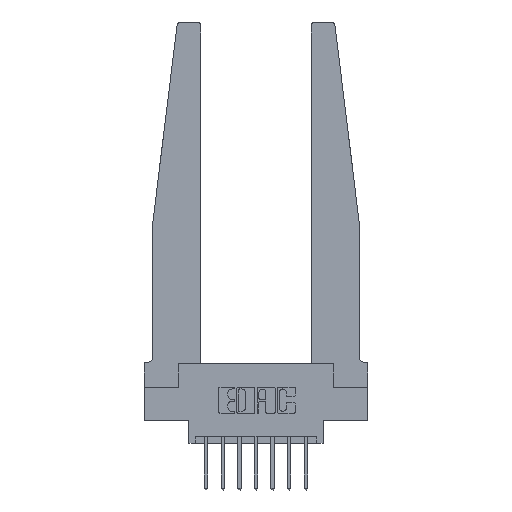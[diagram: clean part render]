
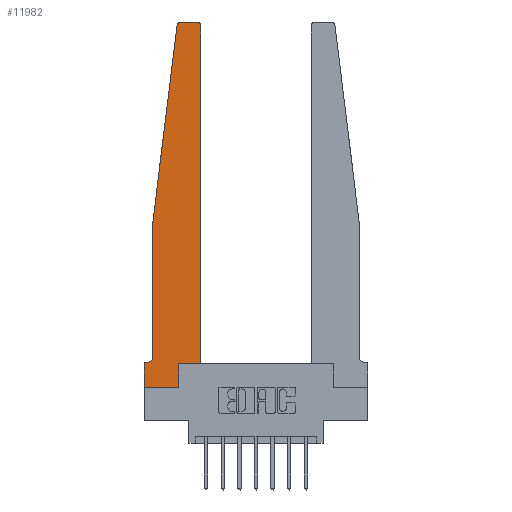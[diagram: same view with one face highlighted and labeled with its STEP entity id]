
A CAD part, top view. The second image highlights one B-rep face of the part: STEP entity #11982.
In plain terms, the highlighted planar face has unit normal (0, 0, 1).
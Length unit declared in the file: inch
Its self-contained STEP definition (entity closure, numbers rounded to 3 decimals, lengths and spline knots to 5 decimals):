
#76 = VERTEX_POINT ( 'NONE', #4507 ) ;
#304 = EDGE_CURVE ( 'NONE', #1373, #2586, #9048, .T. ) ;
#507 = CARTESIAN_POINT ( 'NONE',  ( 0., 0.1875, 0.37 ) ) ;
#565 = ORIENTED_EDGE ( 'NONE', *, *, #2735, .T. ) ;
#770 = CARTESIAN_POINT ( 'NONE',  ( 0.425, 0.18, 0.37 ) ) ;
#789 = LINE ( 'NONE', #14413, #3189 ) ;
#1053 = CARTESIAN_POINT ( 'NONE',  ( 0.065, 0.1875, 0.37 ) ) ;
#1319 = AXIS2_PLACEMENT_3D ( 'NONE', #11494, #12881, #6173 ) ;
#1373 = VERTEX_POINT ( 'NONE', #14378 ) ;
#1492 = EDGE_CURVE ( 'NONE', #8797, #5418, #789, .T. ) ;
#1594 = CARTESIAN_POINT ( 'NONE',  ( 0.2605, 0.18, 0.37 ) ) ;
#1624 = CARTESIAN_POINT ( 'NONE',  ( 0., 0., 0.37 ) ) ;
#1711 = VERTEX_POINT ( 'NONE', #5702 ) ;
#1904 = VECTOR ( 'NONE', #4447, 39.37008 ) ;
#2036 = CARTESIAN_POINT ( 'NONE',  ( 0.395, 2.72, 0.37 ) ) ;
#2131 = EDGE_CURVE ( 'NONE', #6667, #3614, #11939, .T. ) ;
#2146 = LINE ( 'NONE', #7879, #3322 ) ;
#2527 = EDGE_LOOP ( 'NONE', ( #3956, #9566, #7385, #7978, #10287, #3680, #4014, #5228, #5180, #12531, #565, #14125 ) ) ;
#2586 = VERTEX_POINT ( 'NONE', #6468 ) ;
#2670 = CARTESIAN_POINT ( 'NONE',  ( 0.2605, 0.18, 0.37 ) ) ;
#2689 = CARTESIAN_POINT ( 'NONE',  ( 0.015, 0.2375, 0.37 ) ) ;
#2735 = EDGE_CURVE ( 'NONE', #5418, #1373, #2146, .T. ) ;
#2906 = VECTOR ( 'NONE', #9753, 39.37008 ) ;
#2963 = LINE ( 'NONE', #8903, #6334 ) ;
#3189 = VECTOR ( 'NONE', #9775, 39.37008 ) ;
#3256 = VERTEX_POINT ( 'NONE', #13943 ) ;
#3322 = VECTOR ( 'NONE', #12367, 39.37008 ) ;
#3614 = VERTEX_POINT ( 'NONE', #11118 ) ;
#3680 = ORIENTED_EDGE ( 'NONE', *, *, #8718, .T. ) ;
#3815 = AXIS2_PLACEMENT_3D ( 'NONE', #2036, #5167, #5092 ) ;
#3956 = ORIENTED_EDGE ( 'NONE', *, *, #4637, .T. ) ;
#4014 = ORIENTED_EDGE ( 'NONE', *, *, #5359, .T. ) ;
#4137 = VECTOR ( 'NONE', #13999, 39.37008 ) ;
#4188 = CARTESIAN_POINT ( 'NONE',  ( 0.065, 0.2375, 0.37 ) ) ;
#4447 = DIRECTION ( 'NONE',  ( -1., 0., 0. ) ) ;
#4507 = CARTESIAN_POINT ( 'NONE',  ( 0., 0.1875, 0.37 ) ) ;
#4637 = EDGE_CURVE ( 'NONE', #2586, #7283, #12360, .T. ) ;
#5048 = DIRECTION ( 'NONE',  ( 0., 0., 1. ) ) ;
#5092 = DIRECTION ( 'NONE',  ( 1., 0., 0. ) ) ;
#5167 = DIRECTION ( 'NONE',  ( 0., 0., 1. ) ) ;
#5180 = ORIENTED_EDGE ( 'NONE', *, *, #8181, .T. ) ;
#5228 = ORIENTED_EDGE ( 'NONE', *, *, #7321, .T. ) ;
#5359 = EDGE_CURVE ( 'NONE', #76, #1711, #13141, .T. ) ;
#5418 = VERTEX_POINT ( 'NONE', #770 ) ;
#5437 = CARTESIAN_POINT ( 'NONE',  ( 0.2605, 0., 0.37 ) ) ;
#5702 = CARTESIAN_POINT ( 'NONE',  ( 0., 0., 0.37 ) ) ;
#5819 = VERTEX_POINT ( 'NONE', #5437 ) ;
#5835 = VECTOR ( 'NONE', #14401, 39.37008 ) ;
#5953 = CARTESIAN_POINT ( 'NONE',  ( 0.27653, 2.75, 0.37 ) ) ;
#6067 = CIRCLE ( 'NONE', #1319, 0.03 ) ;
#6136 = DIRECTION ( 'NONE',  ( 0., 1., 0. ) ) ;
#6159 = FACE_OUTER_BOUND ( 'NONE', #2527, .T. ) ;
#6173 = DIRECTION ( 'NONE',  ( 1., 0., 0. ) ) ;
#6334 = VECTOR ( 'NONE', #9121, 39.37008 ) ;
#6468 = CARTESIAN_POINT ( 'NONE',  ( 0.395, 2.75, 0.37 ) ) ;
#6667 = VERTEX_POINT ( 'NONE', #4188 ) ;
#6854 = DIRECTION ( 'NONE',  ( -1., 0., 0. ) ) ;
#6862 = DIRECTION ( 'NONE',  ( 1., 0., 0. ) ) ;
#7157 = DIRECTION ( 'NONE',  ( 0., 0., -1. ) ) ;
#7238 = AXIS2_PLACEMENT_3D ( 'NONE', #2689, #7157, #10550 ) ;
#7283 = VERTEX_POINT ( 'NONE', #5953 ) ;
#7321 = EDGE_CURVE ( 'NONE', #1711, #5819, #9347, .T. ) ;
#7385 = ORIENTED_EDGE ( 'NONE', *, *, #11309, .T. ) ;
#7790 = CARTESIAN_POINT ( 'NONE',  ( 0.24675, 2.72367, 0.37 ) ) ;
#7846 = CARTESIAN_POINT ( 'NONE',  ( 0.065, 1.25, 0.37 ) ) ;
#7873 = CARTESIAN_POINT ( 'NONE',  ( 0.25, 2.75, 0.37 ) ) ;
#7879 = CARTESIAN_POINT ( 'NONE',  ( 0.425, 0.18, 0.37 ) ) ;
#7956 = VERTEX_POINT ( 'NONE', #7790 ) ;
#7978 = ORIENTED_EDGE ( 'NONE', *, *, #9094, .T. ) ;
#8181 = EDGE_CURVE ( 'NONE', #5819, #8797, #9240, .T. ) ;
#8718 = EDGE_CURVE ( 'NONE', #3614, #76, #12458, .T. ) ;
#8797 = VERTEX_POINT ( 'NONE', #2670 ) ;
#8903 = CARTESIAN_POINT ( 'NONE',  ( 0.065, 1.25, 0.37 ) ) ;
#9019 = LINE ( 'NONE', #7846, #5835 ) ;
#9048 = CIRCLE ( 'NONE', #3815, 0.03 ) ;
#9094 = EDGE_CURVE ( 'NONE', #3256, #6667, #2963, .T. ) ;
#9121 = DIRECTION ( 'NONE',  ( 0., -1., 0. ) ) ;
#9147 = PLANE ( 'NONE',  #11091 ) ;
#9240 = LINE ( 'NONE', #1594, #9604 ) ;
#9347 = LINE ( 'NONE', #1624, #4137 ) ;
#9566 = ORIENTED_EDGE ( 'NONE', *, *, #10114, .T. ) ;
#9604 = VECTOR ( 'NONE', #6136, 39.37008 ) ;
#9753 = DIRECTION ( 'NONE',  ( 0., -1., 0. ) ) ;
#9775 = DIRECTION ( 'NONE',  ( 1., 0., 0. ) ) ;
#10114 = EDGE_CURVE ( 'NONE', #7283, #7956, #6067, .T. ) ;
#10287 = ORIENTED_EDGE ( 'NONE', *, *, #2131, .T. ) ;
#10550 = DIRECTION ( 'NONE',  ( -1., 0., 0. ) ) ;
#11091 = AXIS2_PLACEMENT_3D ( 'NONE', #507, #5048, #6862 ) ;
#11118 = CARTESIAN_POINT ( 'NONE',  ( 0.015, 0.1875, 0.37 ) ) ;
#11309 = EDGE_CURVE ( 'NONE', #7956, #3256, #9019, .T. ) ;
#11494 = CARTESIAN_POINT ( 'NONE',  ( 0.27653, 2.72, 0.37 ) ) ;
#11939 = CIRCLE ( 'NONE', #7238, 0.05 ) ;
#11977 = VECTOR ( 'NONE', #6854, 39.37008 ) ;
#11982 = ADVANCED_FACE ( 'NONE', ( #6159 ), #9147, .T. ) ;
#12360 = LINE ( 'NONE', #7873, #1904 ) ;
#12367 = DIRECTION ( 'NONE',  ( 0., 1., 0. ) ) ;
#12458 = LINE ( 'NONE', #1053, #11977 ) ;
#12531 = ORIENTED_EDGE ( 'NONE', *, *, #1492, .T. ) ;
#12881 = DIRECTION ( 'NONE',  ( 0., 0., 1. ) ) ;
#13141 = LINE ( 'NONE', #14549, #2906 ) ;
#13943 = CARTESIAN_POINT ( 'NONE',  ( 0.065, 1.25, 0.37 ) ) ;
#13999 = DIRECTION ( 'NONE',  ( 1., 0., 0. ) ) ;
#14125 = ORIENTED_EDGE ( 'NONE', *, *, #304, .T. ) ;
#14378 = CARTESIAN_POINT ( 'NONE',  ( 0.425, 2.72, 0.37 ) ) ;
#14401 = DIRECTION ( 'NONE',  ( -0.122, -0.992, 0. ) ) ;
#14413 = CARTESIAN_POINT ( 'NONE',  ( 0.425, 0.18, 0.37 ) ) ;
#14549 = CARTESIAN_POINT ( 'NONE',  ( 0., 0., 0.37 ) ) ;
